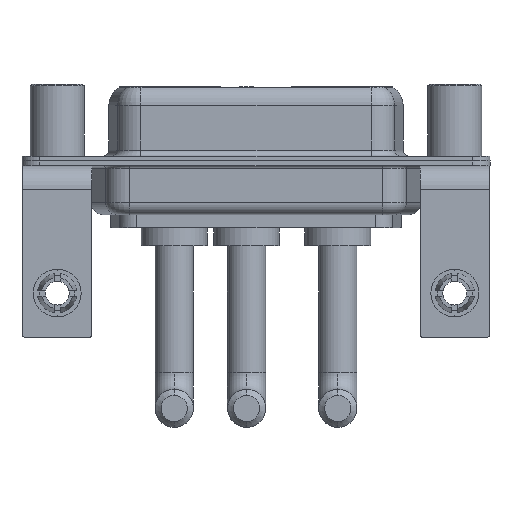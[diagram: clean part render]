
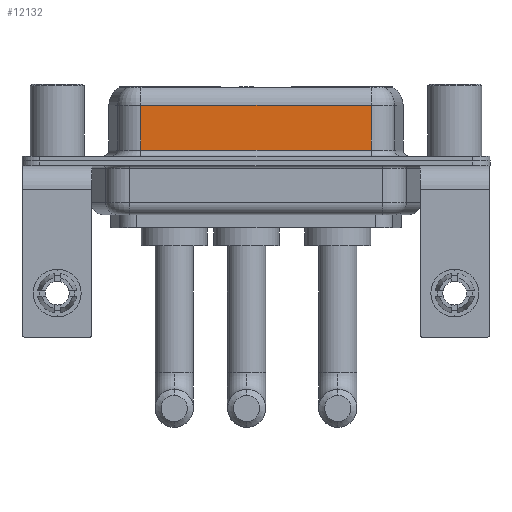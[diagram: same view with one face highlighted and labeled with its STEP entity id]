
A CAD part, front view. The second image highlights one B-rep face of the part: STEP entity #12132.
In plain terms, the highlighted planar face has unit normal (0, -1, 0).
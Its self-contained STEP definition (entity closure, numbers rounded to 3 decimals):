
#65 = VERTEX_POINT ( 'NONE', #10988 ) ;
#688 = DIRECTION ( 'NONE',  ( 0., 0., -1. ) ) ;
#817 = DIRECTION ( 'NONE',  ( 0., 0., -1. ) ) ;
#948 = CARTESIAN_POINT ( 'NONE',  ( 26.287, -3.95, 6.4 ) ) ;
#1637 = EDGE_CURVE ( 'NONE', #65, #7371, #11978, .T. ) ;
#1972 = ORIENTED_EDGE ( 'NONE', *, *, #3267, .T. ) ;
#1980 = CARTESIAN_POINT ( 'NONE',  ( 26.287, -3.95, 6.4 ) ) ;
#2065 = DIRECTION ( 'NONE',  ( 0., 0., 1. ) ) ;
#2185 = VECTOR ( 'NONE', #817, 1000. ) ;
#2516 = VECTOR ( 'NONE', #16632, 1000. ) ;
#3267 = EDGE_CURVE ( 'NONE', #65, #13557, #17907, .T. ) ;
#3909 = LINE ( 'NONE', #14987, #2185 ) ;
#3916 = CARTESIAN_POINT ( 'NONE',  ( 26.287, -3.95, 4.65 ) ) ;
#4246 = EDGE_LOOP ( 'NONE', ( #11106, #1972, #15874, #15417 ) ) ;
#4513 = DIRECTION ( 'NONE',  ( 1., 0., 0. ) ) ;
#6106 = CARTESIAN_POINT ( 'NONE',  ( 26.287, -3.95, 0.9 ) ) ;
#6386 = EDGE_CURVE ( 'NONE', #11188, #7371, #11404, .T. ) ;
#7125 = VECTOR ( 'NONE', #688, 1000. ) ;
#7371 = VERTEX_POINT ( 'NONE', #6106 ) ;
#7517 = CARTESIAN_POINT ( 'NONE',  ( 26.287, -3.95, 0.9 ) ) ;
#8261 = CARTESIAN_POINT ( 'NONE',  ( 7.013, -3.95, 0.9 ) ) ;
#8975 = DIRECTION ( 'NONE',  ( 0., 1., 0. ) ) ;
#9536 = VECTOR ( 'NONE', #4513, 1000. ) ;
#9943 = AXIS2_PLACEMENT_3D ( 'NONE', #1980, #8975, #2065 ) ;
#10332 = PLANE ( 'NONE',  #9943 ) ;
#10988 = CARTESIAN_POINT ( 'NONE',  ( 26.287, -3.95, 4.65 ) ) ;
#11106 = ORIENTED_EDGE ( 'NONE', *, *, #1637, .F. ) ;
#11188 = VERTEX_POINT ( 'NONE', #8261 ) ;
#11404 = LINE ( 'NONE', #7517, #9536 ) ;
#11978 = LINE ( 'NONE', #948, #7125 ) ;
#12132 = ADVANCED_FACE ( 'NONE', ( #13306 ), #10332, .F. ) ;
#13306 = FACE_OUTER_BOUND ( 'NONE', #4246, .T. ) ;
#13557 = VERTEX_POINT ( 'NONE', #16530 ) ;
#14987 = CARTESIAN_POINT ( 'NONE',  ( 7.013, -3.95, 6.4 ) ) ;
#15417 = ORIENTED_EDGE ( 'NONE', *, *, #6386, .T. ) ;
#15874 = ORIENTED_EDGE ( 'NONE', *, *, #16052, .T. ) ;
#16052 = EDGE_CURVE ( 'NONE', #13557, #11188, #3909, .T. ) ;
#16530 = CARTESIAN_POINT ( 'NONE',  ( 7.013, -3.95, 4.65 ) ) ;
#16632 = DIRECTION ( 'NONE',  ( -1., 0., 0. ) ) ;
#17907 = LINE ( 'NONE', #3916, #2516 ) ;
